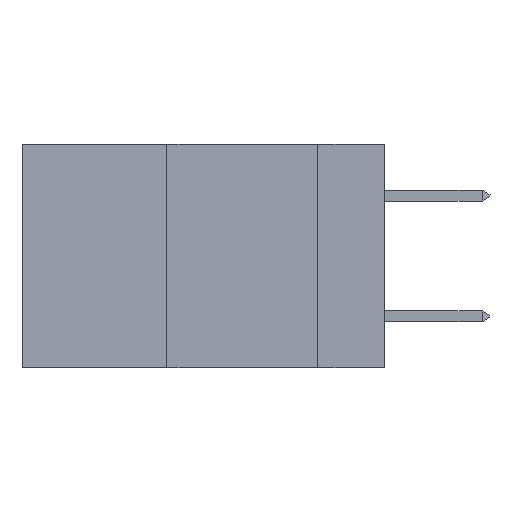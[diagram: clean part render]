
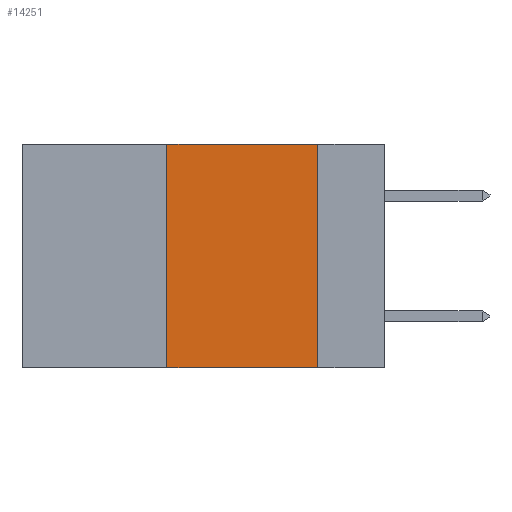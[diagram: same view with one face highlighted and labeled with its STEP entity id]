
A CAD part, left-side view. The second image highlights one B-rep face of the part: STEP entity #14251.
In plain terms, the highlighted planar face has unit normal (-1, 0, 0).
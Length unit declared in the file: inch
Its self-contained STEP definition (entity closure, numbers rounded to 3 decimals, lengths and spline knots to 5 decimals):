
#70 = ORIENTED_EDGE ( 'NONE', *, *, #15043, .F. ) ;
#82 = VECTOR ( 'NONE', #16825, 39.37008 ) ;
#164 = VECTOR ( 'NONE', #1758, 39.37008 ) ;
#684 = FACE_OUTER_BOUND ( 'NONE', #3909, .T. ) ;
#1633 = VECTOR ( 'NONE', #13791, 39.37008 ) ;
#1758 = DIRECTION ( 'NONE',  ( 0., 0., 1. ) ) ;
#3199 = ORIENTED_EDGE ( 'NONE', *, *, #8068, .F. ) ;
#3484 = CARTESIAN_POINT ( 'NONE',  ( 0., 0.6, 0. ) ) ;
#3707 = LINE ( 'NONE', #9788, #1633 ) ;
#3909 = EDGE_LOOP ( 'NONE', ( #70, #6507, #3199, #16410 ) ) ;
#5292 = CARTESIAN_POINT ( 'NONE',  ( 0., 0.11, -0.37 ) ) ;
#5778 = CARTESIAN_POINT ( 'NONE',  ( 0., 0.11, 0. ) ) ;
#5959 = CARTESIAN_POINT ( 'NONE',  ( 0., 0.6, 0. ) ) ;
#6507 = ORIENTED_EDGE ( 'NONE', *, *, #7664, .F. ) ;
#7201 = AXIS2_PLACEMENT_3D ( 'NONE', #5959, #12368, #7280 ) ;
#7280 = DIRECTION ( 'NONE',  ( 0., 0., -1. ) ) ;
#7532 = VERTEX_POINT ( 'NONE', #8390 ) ;
#7664 = EDGE_CURVE ( 'NONE', #7532, #16622, #9984, .T. ) ;
#8068 = EDGE_CURVE ( 'NONE', #15246, #7532, #8345, .T. ) ;
#8345 = LINE ( 'NONE', #16199, #164 ) ;
#8390 = CARTESIAN_POINT ( 'NONE',  ( 0., 0.36, 0. ) ) ;
#8533 = PLANE ( 'NONE',  #7201 ) ;
#9788 = CARTESIAN_POINT ( 'NONE',  ( 0., 0.11, 0. ) ) ;
#9962 = CARTESIAN_POINT ( 'NONE',  ( 0., 0.36, -0.37 ) ) ;
#9984 = LINE ( 'NONE', #3484, #12490 ) ;
#10492 = VERTEX_POINT ( 'NONE', #5292 ) ;
#11327 = DIRECTION ( 'NONE',  ( 0., -1., 0. ) ) ;
#12368 = DIRECTION ( 'NONE',  ( 1., 0., 0. ) ) ;
#12490 = VECTOR ( 'NONE', #11327, 39.37008 ) ;
#12974 = CARTESIAN_POINT ( 'NONE',  ( 0., 0.6, -0.37 ) ) ;
#13791 = DIRECTION ( 'NONE',  ( 0., 0., -1. ) ) ;
#14139 = EDGE_CURVE ( 'NONE', #15246, #10492, #15917, .T. ) ;
#14251 = ADVANCED_FACE ( 'NONE', ( #684 ), #8533, .F. ) ;
#15043 = EDGE_CURVE ( 'NONE', #16622, #10492, #3707, .T. ) ;
#15246 = VERTEX_POINT ( 'NONE', #9962 ) ;
#15917 = LINE ( 'NONE', #12974, #82 ) ;
#16199 = CARTESIAN_POINT ( 'NONE',  ( 0., 0.36, 0. ) ) ;
#16410 = ORIENTED_EDGE ( 'NONE', *, *, #14139, .T. ) ;
#16622 = VERTEX_POINT ( 'NONE', #5778 ) ;
#16825 = DIRECTION ( 'NONE',  ( 0., -1., 0. ) ) ;
